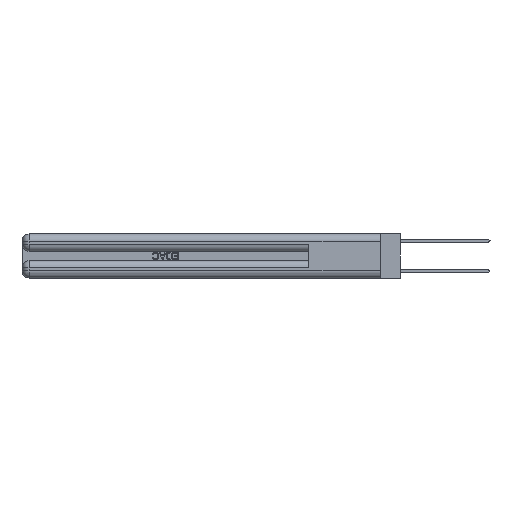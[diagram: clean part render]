
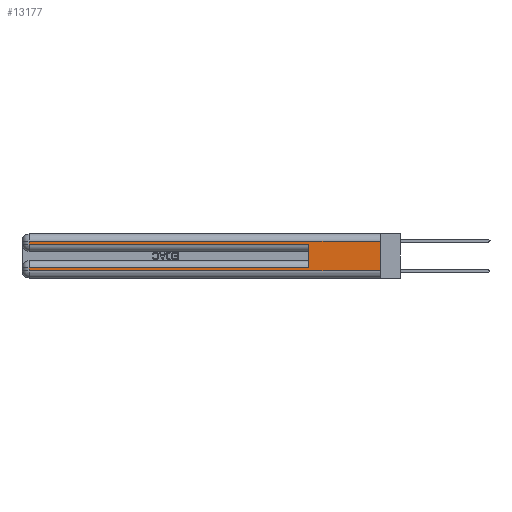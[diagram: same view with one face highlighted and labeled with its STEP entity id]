
A CAD part, left-side view. The second image highlights one B-rep face of the part: STEP entity #13177.
In plain terms, the highlighted planar face has unit normal (-1, 0, 0).
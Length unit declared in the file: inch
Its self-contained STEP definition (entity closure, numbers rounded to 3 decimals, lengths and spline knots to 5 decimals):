
#219 = ORIENTED_EDGE ( 'NONE', *, *, #10445, .T. ) ;
#342 = ORIENTED_EDGE ( 'NONE', *, *, #29100, .F. ) ;
#396 = CARTESIAN_POINT ( 'NONE',  ( 0., 0., 0.06 ) ) ;
#1200 = DIRECTION ( 'NONE',  ( 0., 0., 1. ) ) ;
#1321 = CARTESIAN_POINT ( 'NONE',  ( 0., 0., 0.37 ) ) ;
#2566 = CARTESIAN_POINT ( 'NONE',  ( 0., 0., 0.06 ) ) ;
#2795 = EDGE_LOOP ( 'NONE', ( #9017, #16574, #7655, #219, #342, #9144, #10211, #4012 ) ) ;
#2855 = DIRECTION ( 'NONE',  ( 0., -1., 0. ) ) ;
#2986 = CARTESIAN_POINT ( 'NONE',  ( 0., 0.6, 0.285 ) ) ;
#3225 = LINE ( 'NONE', #17485, #14752 ) ;
#3625 = LINE ( 'NONE', #18389, #21670 ) ;
#3662 = CARTESIAN_POINT ( 'NONE',  ( 0., 2.94, 0.085 ) ) ;
#3895 = AXIS2_PLACEMENT_3D ( 'NONE', #12842, #25138, #10469 ) ;
#4012 = ORIENTED_EDGE ( 'NONE', *, *, #16013, .T. ) ;
#4107 = LINE ( 'NONE', #18230, #9120 ) ;
#4372 = CARTESIAN_POINT ( 'NONE',  ( 0., 2.94, 0.285 ) ) ;
#4502 = DIRECTION ( 'NONE',  ( 0., 0., -1. ) ) ;
#6380 = VECTOR ( 'NONE', #4502, 39.37008 ) ;
#7655 = ORIENTED_EDGE ( 'NONE', *, *, #12092, .T. ) ;
#7715 = CARTESIAN_POINT ( 'NONE',  ( 0., 2.94, 0.31 ) ) ;
#7974 = PLANE ( 'NONE',  #3895 ) ;
#9017 = ORIENTED_EDGE ( 'NONE', *, *, #18695, .F. ) ;
#9120 = VECTOR ( 'NONE', #20670, 39.37008 ) ;
#9144 = ORIENTED_EDGE ( 'NONE', *, *, #27446, .T. ) ;
#10211 = ORIENTED_EDGE ( 'NONE', *, *, #20929, .T. ) ;
#10445 = EDGE_CURVE ( 'NONE', #17734, #29591, #3225, .T. ) ;
#10469 = DIRECTION ( 'NONE',  ( 0., 0., -1. ) ) ;
#11098 = DIRECTION ( 'NONE',  ( 0., 0., -1. ) ) ;
#11396 = VERTEX_POINT ( 'NONE', #28226 ) ;
#11938 = CARTESIAN_POINT ( 'NONE',  ( 0., 0., 0.31 ) ) ;
#12092 = EDGE_CURVE ( 'NONE', #24819, #17734, #26727, .T. ) ;
#12328 = LINE ( 'NONE', #11938, #24581 ) ;
#12842 = CARTESIAN_POINT ( 'NONE',  ( 0., 0., 0.37 ) ) ;
#13114 = VERTEX_POINT ( 'NONE', #15412 ) ;
#13177 = ADVANCED_FACE ( 'NONE', ( #15599 ), #7974, .F. ) ;
#13509 = LINE ( 'NONE', #396, #25747 ) ;
#14406 = DIRECTION ( 'NONE',  ( 0., 1., 0. ) ) ;
#14752 = VECTOR ( 'NONE', #19931, 39.37008 ) ;
#15412 = CARTESIAN_POINT ( 'NONE',  ( 0., 0.6, 0.085 ) ) ;
#15599 = FACE_OUTER_BOUND ( 'NONE', #2795, .T. ) ;
#16013 = EDGE_CURVE ( 'NONE', #16819, #24753, #13509, .T. ) ;
#16574 = ORIENTED_EDGE ( 'NONE', *, *, #17032, .T. ) ;
#16819 = VERTEX_POINT ( 'NONE', #18077 ) ;
#17032 = EDGE_CURVE ( 'NONE', #11396, #24819, #12328, .T. ) ;
#17485 = CARTESIAN_POINT ( 'NONE',  ( 0., 0., 0.285 ) ) ;
#17734 = VERTEX_POINT ( 'NONE', #4372 ) ;
#18077 = CARTESIAN_POINT ( 'NONE',  ( 0., 2.94, 0.06 ) ) ;
#18230 = CARTESIAN_POINT ( 'NONE',  ( 0., 0., 0.085 ) ) ;
#18389 = CARTESIAN_POINT ( 'NONE',  ( 0., 0.6, 0.145 ) ) ;
#18695 = EDGE_CURVE ( 'NONE', #11396, #24753, #28389, .T. ) ;
#19931 = DIRECTION ( 'NONE',  ( 0., -1., 0. ) ) ;
#20186 = LINE ( 'NONE', #24040, #6380 ) ;
#20670 = DIRECTION ( 'NONE',  ( 0., 1., 0. ) ) ;
#20684 = VERTEX_POINT ( 'NONE', #3662 ) ;
#20929 = EDGE_CURVE ( 'NONE', #20684, #16819, #20186, .T. ) ;
#21129 = VECTOR ( 'NONE', #11098, 39.37008 ) ;
#21142 = DIRECTION ( 'NONE',  ( 0., 0., -1. ) ) ;
#21670 = VECTOR ( 'NONE', #1200, 39.37008 ) ;
#24040 = CARTESIAN_POINT ( 'NONE',  ( 0., 2.94, 0.37 ) ) ;
#24581 = VECTOR ( 'NONE', #14406, 39.37008 ) ;
#24753 = VERTEX_POINT ( 'NONE', #2566 ) ;
#24819 = VERTEX_POINT ( 'NONE', #7715 ) ;
#25138 = DIRECTION ( 'NONE',  ( 1., 0., 0. ) ) ;
#25747 = VECTOR ( 'NONE', #2855, 39.37008 ) ;
#25981 = VECTOR ( 'NONE', #21142, 39.37008 ) ;
#26037 = CARTESIAN_POINT ( 'NONE',  ( 0., 2.94, 0.37 ) ) ;
#26727 = LINE ( 'NONE', #26037, #25981 ) ;
#27446 = EDGE_CURVE ( 'NONE', #13114, #20684, #4107, .T. ) ;
#28226 = CARTESIAN_POINT ( 'NONE',  ( 0., 0., 0.31 ) ) ;
#28389 = LINE ( 'NONE', #1321, #21129 ) ;
#29100 = EDGE_CURVE ( 'NONE', #13114, #29591, #3625, .T. ) ;
#29591 = VERTEX_POINT ( 'NONE', #2986 ) ;
